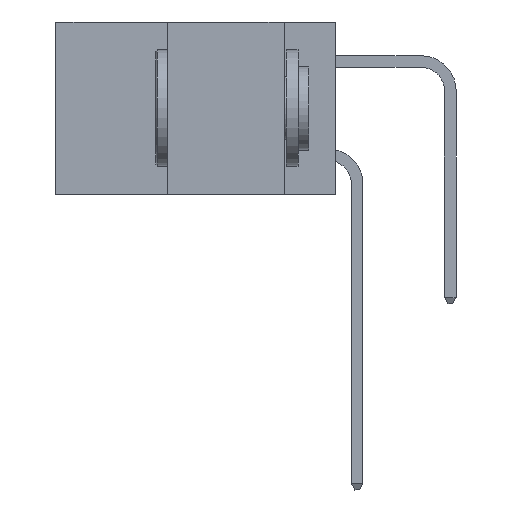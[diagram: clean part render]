
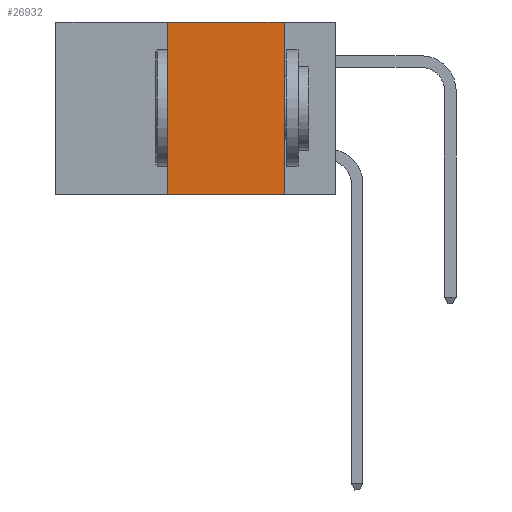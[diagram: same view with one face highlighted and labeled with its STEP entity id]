
A CAD part, left-side view. The second image highlights one B-rep face of the part: STEP entity #26932.
In plain terms, the highlighted planar face has unit normal (-1, 0, 0).
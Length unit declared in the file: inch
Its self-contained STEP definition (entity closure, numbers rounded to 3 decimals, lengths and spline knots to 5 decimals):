
#111 = ORIENTED_EDGE ( 'NONE', *, *, #11188, .F. ) ;
#528 = VERTEX_POINT ( 'NONE', #9719 ) ;
#603 = PLANE ( 'NONE',  #25333 ) ;
#697 = CARTESIAN_POINT ( 'NONE',  ( 0., 0.36, 0. ) ) ;
#1744 = ORIENTED_EDGE ( 'NONE', *, *, #13365, .F. ) ;
#1834 = LINE ( 'NONE', #697, #27534 ) ;
#1865 = CARTESIAN_POINT ( 'NONE',  ( 0., 0.6, 0. ) ) ;
#1933 = CARTESIAN_POINT ( 'NONE',  ( 0., 0.36, -0.37 ) ) ;
#2116 = VERTEX_POINT ( 'NONE', #8463 ) ;
#3420 = LINE ( 'NONE', #21719, #26945 ) ;
#4670 = LINE ( 'NONE', #14331, #16431 ) ;
#4797 = EDGE_CURVE ( 'NONE', #528, #26240, #15760, .T. ) ;
#5014 = CARTESIAN_POINT ( 'NONE',  ( 0., 0.11, -0.37 ) ) ;
#6456 = DIRECTION ( 'NONE',  ( 1., 0., 0. ) ) ;
#8463 = CARTESIAN_POINT ( 'NONE',  ( 0., 0.36, 0. ) ) ;
#9719 = CARTESIAN_POINT ( 'NONE',  ( 0., 0.11, 0. ) ) ;
#10132 = CARTESIAN_POINT ( 'NONE',  ( 0., 0.11, 0. ) ) ;
#11188 = EDGE_CURVE ( 'NONE', #19097, #2116, #1834, .T. ) ;
#13365 = EDGE_CURVE ( 'NONE', #2116, #528, #3420, .T. ) ;
#14331 = CARTESIAN_POINT ( 'NONE',  ( 0., 0.6, -0.37 ) ) ;
#14613 = FACE_OUTER_BOUND ( 'NONE', #18799, .T. ) ;
#14901 = ORIENTED_EDGE ( 'NONE', *, *, #4797, .F. ) ;
#14932 = DIRECTION ( 'NONE',  ( 0., 0., -1. ) ) ;
#15760 = LINE ( 'NONE', #10132, #23322 ) ;
#16431 = VECTOR ( 'NONE', #16511, 39.37008 ) ;
#16511 = DIRECTION ( 'NONE',  ( 0., -1., 0. ) ) ;
#17053 = DIRECTION ( 'NONE',  ( 0., 0., 1. ) ) ;
#18799 = EDGE_LOOP ( 'NONE', ( #14901, #1744, #111, #19833 ) ) ;
#19097 = VERTEX_POINT ( 'NONE', #1933 ) ;
#19833 = ORIENTED_EDGE ( 'NONE', *, *, #25879, .T. ) ;
#21719 = CARTESIAN_POINT ( 'NONE',  ( 0., 0.6, 0. ) ) ;
#23322 = VECTOR ( 'NONE', #14932, 39.37008 ) ;
#24002 = DIRECTION ( 'NONE',  ( 0., -1., 0. ) ) ;
#24717 = DIRECTION ( 'NONE',  ( 0., 0., -1. ) ) ;
#25333 = AXIS2_PLACEMENT_3D ( 'NONE', #1865, #6456, #24717 ) ;
#25879 = EDGE_CURVE ( 'NONE', #19097, #26240, #4670, .T. ) ;
#26240 = VERTEX_POINT ( 'NONE', #5014 ) ;
#26932 = ADVANCED_FACE ( 'NONE', ( #14613 ), #603, .F. ) ;
#26945 = VECTOR ( 'NONE', #24002, 39.37008 ) ;
#27534 = VECTOR ( 'NONE', #17053, 39.37008 ) ;
